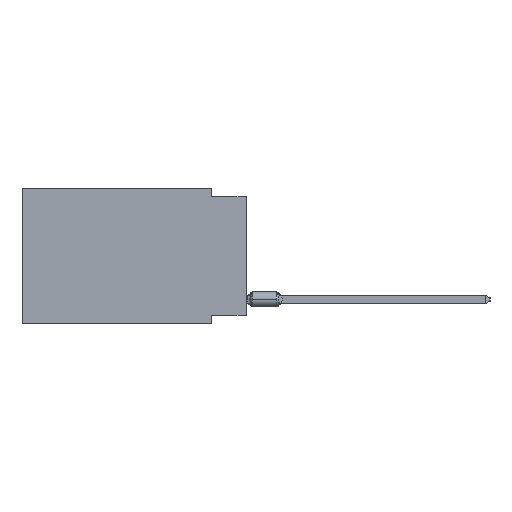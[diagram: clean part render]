
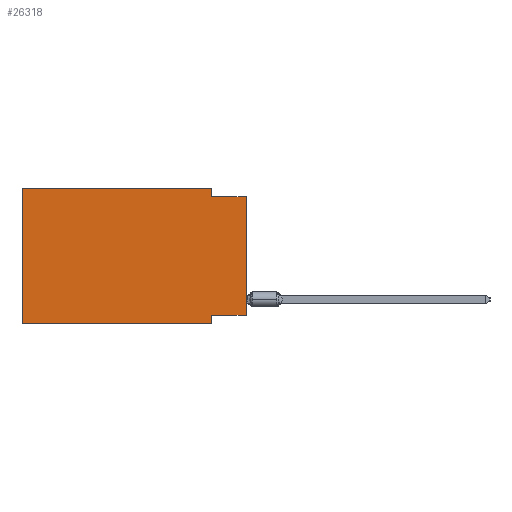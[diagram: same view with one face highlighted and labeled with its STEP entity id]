
A CAD part, left-side view. The second image highlights one B-rep face of the part: STEP entity #26318.
In plain terms, the highlighted planar face has unit normal (-1, 0, 0).
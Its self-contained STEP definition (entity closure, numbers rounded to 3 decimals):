
#101 = CARTESIAN_POINT ( 'NONE',  ( 0., 2.54, -9.271 ) ) ;
#380 = VECTOR ( 'NONE', #1251, 1000. ) ;
#675 = CARTESIAN_POINT ( 'NONE',  ( 0., 0., 0. ) ) ;
#1251 = DIRECTION ( 'NONE',  ( 0., 0., 1. ) ) ;
#2794 = CARTESIAN_POINT ( 'NONE',  ( 0., 2.54, 0. ) ) ;
#2866 = ORIENTED_EDGE ( 'NONE', *, *, #25286, .F. ) ;
#4134 = EDGE_CURVE ( 'NONE', #30291, #12464, #33399, .T. ) ;
#4484 = VECTOR ( 'NONE', #39535, 1000. ) ;
#4779 = VERTEX_POINT ( 'NONE', #101 ) ;
#6484 = VERTEX_POINT ( 'NONE', #47176 ) ;
#6818 = CARTESIAN_POINT ( 'NONE',  ( 0., 0., -9.271 ) ) ;
#7371 = LINE ( 'NONE', #6818, #50296 ) ;
#7924 = DIRECTION ( 'NONE',  ( 0., 1., 0. ) ) ;
#8430 = CARTESIAN_POINT ( 'NONE',  ( 0., 16.383, 0. ) ) ;
#9199 = CARTESIAN_POINT ( 'NONE',  ( 0., 2.54, -9.906 ) ) ;
#9310 = EDGE_CURVE ( 'NONE', #6484, #30291, #10076, .T. ) ;
#10076 = LINE ( 'NONE', #49000, #35820 ) ;
#11803 = VERTEX_POINT ( 'NONE', #15849 ) ;
#12464 = VERTEX_POINT ( 'NONE', #24776 ) ;
#14128 = CARTESIAN_POINT ( 'NONE',  ( 0., 16.383, 0. ) ) ;
#15849 = CARTESIAN_POINT ( 'NONE',  ( 0., 16.383, -9.906 ) ) ;
#17513 = LINE ( 'NONE', #34960, #4484 ) ;
#18872 = VECTOR ( 'NONE', #55175, 1000. ) ;
#19104 = ORIENTED_EDGE ( 'NONE', *, *, #25316, .T. ) ;
#19377 = EDGE_CURVE ( 'NONE', #12464, #53706, #17513, .T. ) ;
#20305 = CARTESIAN_POINT ( 'NONE',  ( 0., 2.54, -9.906 ) ) ;
#24776 = CARTESIAN_POINT ( 'NONE',  ( 0., 2.54, -0.635 ) ) ;
#24869 = DIRECTION ( 'NONE',  ( 0., 0., -1. ) ) ;
#24897 = CARTESIAN_POINT ( 'NONE',  ( 0., 2.54, 0. ) ) ;
#25024 = VECTOR ( 'NONE', #38770, 1000. ) ;
#25072 = EDGE_CURVE ( 'NONE', #11803, #48301, #30735, .T. ) ;
#25286 = EDGE_CURVE ( 'NONE', #11803, #6484, #49617, .T. ) ;
#25316 = EDGE_CURVE ( 'NONE', #25764, #53706, #40446, .T. ) ;
#25764 = VERTEX_POINT ( 'NONE', #28932 ) ;
#26318 = ADVANCED_FACE ( 'NONE', ( #30188 ), #47644, .F. ) ;
#26452 = CARTESIAN_POINT ( 'NONE',  ( 0., 16.383, -9.906 ) ) ;
#27250 = DIRECTION ( 'NONE',  ( 0., -1., 0. ) ) ;
#28903 = LINE ( 'NONE', #20305, #38732 ) ;
#28932 = CARTESIAN_POINT ( 'NONE',  ( 0., 0., -9.271 ) ) ;
#29548 = ORIENTED_EDGE ( 'NONE', *, *, #25072, .T. ) ;
#30188 = FACE_OUTER_BOUND ( 'NONE', #35461, .T. ) ;
#30291 = VERTEX_POINT ( 'NONE', #24897 ) ;
#30735 = LINE ( 'NONE', #26452, #25024 ) ;
#33274 = VECTOR ( 'NONE', #48762, 1000. ) ;
#33399 = LINE ( 'NONE', #2794, #18872 ) ;
#34200 = DIRECTION ( 'NONE',  ( 0., 0., -1. ) ) ;
#34750 = DIRECTION ( 'NONE',  ( 1., 0., 0. ) ) ;
#34960 = CARTESIAN_POINT ( 'NONE',  ( 0., 0., -0.635 ) ) ;
#35461 = EDGE_LOOP ( 'NONE', ( #19104, #42324, #41413, #42089, #2866, #29548, #48648, #49499 ) ) ;
#35820 = VECTOR ( 'NONE', #27250, 1000. ) ;
#36993 = AXIS2_PLACEMENT_3D ( 'NONE', #8430, #34750, #34200 ) ;
#38732 = VECTOR ( 'NONE', #24869, 1000. ) ;
#38770 = DIRECTION ( 'NONE',  ( 0., -1., 0. ) ) ;
#39535 = DIRECTION ( 'NONE',  ( 0., -1., 0. ) ) ;
#40446 = LINE ( 'NONE', #675, #33274 ) ;
#41413 = ORIENTED_EDGE ( 'NONE', *, *, #4134, .F. ) ;
#42089 = ORIENTED_EDGE ( 'NONE', *, *, #9310, .F. ) ;
#42324 = ORIENTED_EDGE ( 'NONE', *, *, #19377, .F. ) ;
#42839 = EDGE_CURVE ( 'NONE', #4779, #48301, #28903, .T. ) ;
#47176 = CARTESIAN_POINT ( 'NONE',  ( 0., 16.383, 0. ) ) ;
#47644 = PLANE ( 'NONE',  #36993 ) ;
#48301 = VERTEX_POINT ( 'NONE', #9199 ) ;
#48648 = ORIENTED_EDGE ( 'NONE', *, *, #42839, .F. ) ;
#48762 = DIRECTION ( 'NONE',  ( 0., 0., 1. ) ) ;
#49000 = CARTESIAN_POINT ( 'NONE',  ( 0., 16.383, 0. ) ) ;
#49499 = ORIENTED_EDGE ( 'NONE', *, *, #54918, .F. ) ;
#49617 = LINE ( 'NONE', #14128, #380 ) ;
#50296 = VECTOR ( 'NONE', #7924, 1000. ) ;
#52266 = CARTESIAN_POINT ( 'NONE',  ( 0., 0., -0.635 ) ) ;
#53706 = VERTEX_POINT ( 'NONE', #52266 ) ;
#54918 = EDGE_CURVE ( 'NONE', #25764, #4779, #7371, .T. ) ;
#55175 = DIRECTION ( 'NONE',  ( 0., 0., -1. ) ) ;
